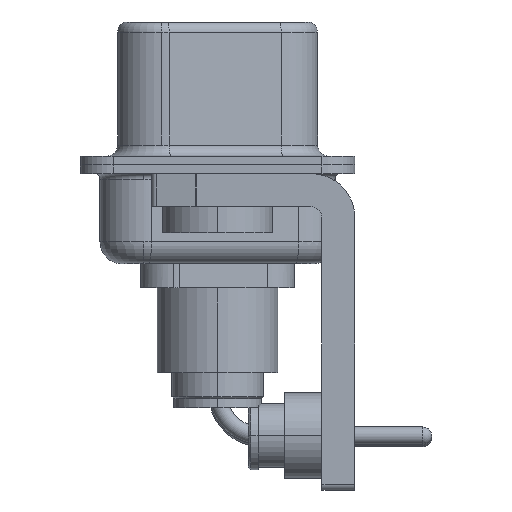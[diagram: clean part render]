
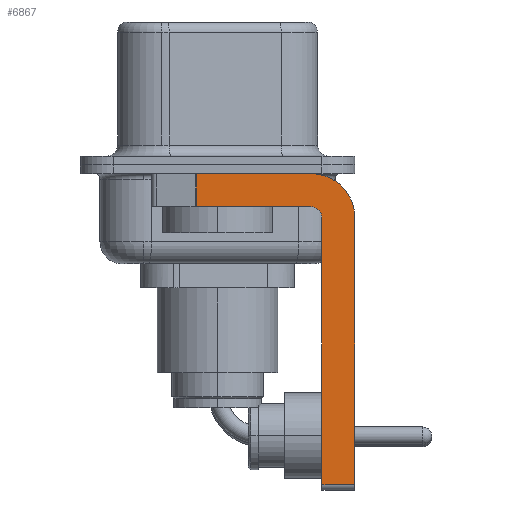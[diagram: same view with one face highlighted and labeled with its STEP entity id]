
A CAD part, left-side view. The second image highlights one B-rep face of the part: STEP entity #6867.
In plain terms, the highlighted planar face has unit normal (-1, 0, 0).
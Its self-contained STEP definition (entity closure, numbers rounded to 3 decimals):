
#140 = DIRECTION ( 'NONE',  ( 0., 0., -1. ) ) ;
#364 = VERTEX_POINT ( 'NONE', #16536 ) ;
#411 = CARTESIAN_POINT ( 'NONE',  ( -2.9, 0.978, -1.9 ) ) ;
#670 = LINE ( 'NONE', #19739, #9148 ) ;
#1007 = PLANE ( 'NONE',  #2094 ) ;
#1545 = EDGE_LOOP ( 'NONE', ( #10184, #13130, #2830, #17559, #5367, #2403, #8620, #9179 ) ) ;
#1647 = LINE ( 'NONE', #20496, #19744 ) ;
#1944 = EDGE_CURVE ( 'NONE', #18033, #9209, #670, .T. ) ;
#2094 = AXIS2_PLACEMENT_3D ( 'NONE', #13612, #19861, #5459 ) ;
#2172 = AXIS2_PLACEMENT_3D ( 'NONE', #6543, #6442, #9485 ) ;
#2274 = VECTOR ( 'NONE', #10364, 1000. ) ;
#2403 = ORIENTED_EDGE ( 'NONE', *, *, #13977, .T. ) ;
#2830 = ORIENTED_EDGE ( 'NONE', *, *, #20082, .F. ) ;
#2891 = CIRCLE ( 'NONE', #14627, 2. ) ;
#2917 = CARTESIAN_POINT ( 'NONE',  ( -2.9, -6.25, -2.4 ) ) ;
#3741 = DIRECTION ( 'NONE',  ( 0., 0., -1. ) ) ;
#4325 = LINE ( 'NONE', #13971, #19438 ) ;
#4402 = EDGE_CURVE ( 'NONE', #364, #16126, #4325, .T. ) ;
#4829 = CARTESIAN_POINT ( 'NONE',  ( -2.9, -4.25, -1.9 ) ) ;
#5367 = ORIENTED_EDGE ( 'NONE', *, *, #14079, .F. ) ;
#5459 = DIRECTION ( 'NONE',  ( 0., 0., -1. ) ) ;
#5527 = CIRCLE ( 'NONE', #2172, 0.5 ) ;
#5602 = EDGE_CURVE ( 'NONE', #16126, #18033, #2891, .T. ) ;
#5960 = LINE ( 'NONE', #10768, #2274 ) ;
#6442 = DIRECTION ( 'NONE',  ( -1., 0., 0. ) ) ;
#6533 = VERTEX_POINT ( 'NONE', #19029 ) ;
#6543 = CARTESIAN_POINT ( 'NONE',  ( -2.9, -4.25, -2.4 ) ) ;
#6867 = ADVANCED_FACE ( 'NONE', ( #7212 ), #1007, .F. ) ;
#7105 = VECTOR ( 'NONE', #9436, 1000. ) ;
#7212 = FACE_OUTER_BOUND ( 'NONE', #1545, .T. ) ;
#7934 = CARTESIAN_POINT ( 'NONE',  ( -2.9, 0.978, -1.9 ) ) ;
#8620 = ORIENTED_EDGE ( 'NONE', *, *, #1944, .F. ) ;
#9148 = VECTOR ( 'NONE', #3741, 1000. ) ;
#9179 = ORIENTED_EDGE ( 'NONE', *, *, #5602, .F. ) ;
#9209 = VERTEX_POINT ( 'NONE', #17870 ) ;
#9436 = DIRECTION ( 'NONE',  ( 0., 1., 0. ) ) ;
#9485 = DIRECTION ( 'NONE',  ( 0., 0., 1. ) ) ;
#9515 = CARTESIAN_POINT ( 'NONE',  ( -2.9, -4.25, -2.4 ) ) ;
#10184 = ORIENTED_EDGE ( 'NONE', *, *, #4402, .F. ) ;
#10364 = DIRECTION ( 'NONE',  ( 0., -1., 0. ) ) ;
#10756 = EDGE_CURVE ( 'NONE', #13638, #6533, #5527, .T. ) ;
#10768 = CARTESIAN_POINT ( 'NONE',  ( -2.9, -4.25, -14.55 ) ) ;
#11282 = CARTESIAN_POINT ( 'NONE',  ( -2.9, -4.75, -14.55 ) ) ;
#11305 = LINE ( 'NONE', #4829, #7105 ) ;
#12148 = VERTEX_POINT ( 'NONE', #11282 ) ;
#12684 = CARTESIAN_POINT ( 'NONE',  ( -2.9, -4.75, -2.4 ) ) ;
#12752 = VECTOR ( 'NONE', #140, 1000. ) ;
#13130 = ORIENTED_EDGE ( 'NONE', *, *, #18705, .T. ) ;
#13612 = CARTESIAN_POINT ( 'NONE',  ( -2.9, -4.25, -2.4 ) ) ;
#13638 = VERTEX_POINT ( 'NONE', #12684 ) ;
#13658 = DIRECTION ( 'NONE',  ( 0., -1., 0. ) ) ;
#13971 = CARTESIAN_POINT ( 'NONE',  ( -2.9, 3., -0.4 ) ) ;
#13977 = EDGE_CURVE ( 'NONE', #12148, #9209, #5960, .T. ) ;
#14079 = EDGE_CURVE ( 'NONE', #12148, #13638, #1647, .T. ) ;
#14627 = AXIS2_PLACEMENT_3D ( 'NONE', #9515, #15931, #17216 ) ;
#15821 = LINE ( 'NONE', #7934, #12752 ) ;
#15931 = DIRECTION ( 'NONE',  ( 1., 0., 0. ) ) ;
#16126 = VERTEX_POINT ( 'NONE', #16644 ) ;
#16536 = CARTESIAN_POINT ( 'NONE',  ( -2.9, 0.978, -0.4 ) ) ;
#16644 = CARTESIAN_POINT ( 'NONE',  ( -2.9, -4.25, -0.4 ) ) ;
#17216 = DIRECTION ( 'NONE',  ( 0., 0., -1. ) ) ;
#17559 = ORIENTED_EDGE ( 'NONE', *, *, #10756, .F. ) ;
#17870 = CARTESIAN_POINT ( 'NONE',  ( -2.9, -6.25, -14.55 ) ) ;
#18033 = VERTEX_POINT ( 'NONE', #2917 ) ;
#18705 = EDGE_CURVE ( 'NONE', #364, #19740, #15821, .T. ) ;
#19029 = CARTESIAN_POINT ( 'NONE',  ( -2.9, -4.25, -1.9 ) ) ;
#19214 = DIRECTION ( 'NONE',  ( 0., 0., 1. ) ) ;
#19438 = VECTOR ( 'NONE', #13658, 1000. ) ;
#19739 = CARTESIAN_POINT ( 'NONE',  ( -2.9, -6.25, -2.4 ) ) ;
#19740 = VERTEX_POINT ( 'NONE', #411 ) ;
#19744 = VECTOR ( 'NONE', #19214, 1000. ) ;
#19861 = DIRECTION ( 'NONE',  ( 1., 0., 0. ) ) ;
#20082 = EDGE_CURVE ( 'NONE', #6533, #19740, #11305, .T. ) ;
#20496 = CARTESIAN_POINT ( 'NONE',  ( -2.9, -4.75, -14.8 ) ) ;
